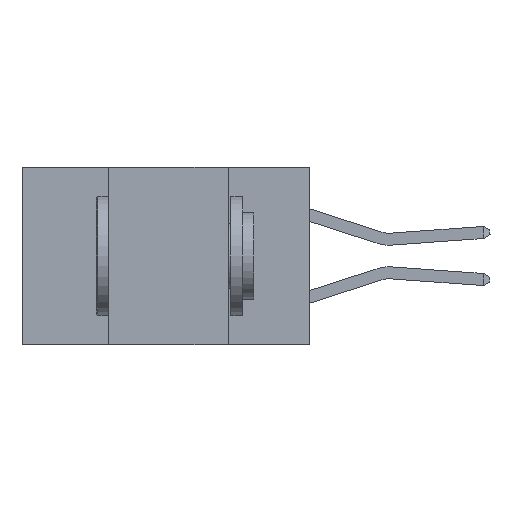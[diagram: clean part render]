
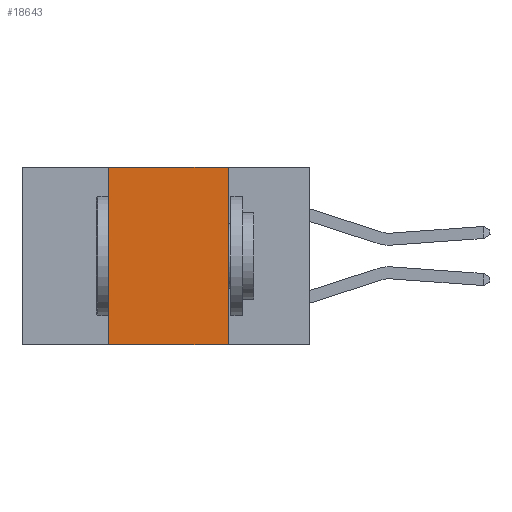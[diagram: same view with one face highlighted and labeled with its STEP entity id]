
A CAD part, left-side view. The second image highlights one B-rep face of the part: STEP entity #18643.
In plain terms, the highlighted planar face has unit normal (-1, 0, 0).
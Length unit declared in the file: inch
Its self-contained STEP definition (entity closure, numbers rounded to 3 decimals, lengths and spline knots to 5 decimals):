
#497 = ORIENTED_EDGE ( 'NONE', *, *, #518, .F. ) ;
#518 = EDGE_CURVE ( 'NONE', #4968, #32732, #17032, .T. ) ;
#2353 = DIRECTION ( 'NONE',  ( 0., 0., -1. ) ) ;
#3965 = VECTOR ( 'NONE', #21358, 39.37008 ) ;
#4008 = EDGE_LOOP ( 'NONE', ( #28634, #497, #12691, #19576 ) ) ;
#4880 = CARTESIAN_POINT ( 'NONE',  ( 0., 0.17, 0. ) ) ;
#4968 = VERTEX_POINT ( 'NONE', #7641 ) ;
#5477 = EDGE_CURVE ( 'NONE', #16546, #4968, #24259, .T. ) ;
#7457 = DIRECTION ( 'NONE',  ( 0., 0., -1. ) ) ;
#7641 = CARTESIAN_POINT ( 'NONE',  ( 0., 0.42, 0. ) ) ;
#9097 = DIRECTION ( 'NONE',  ( 0., -1., 0. ) ) ;
#11531 = FACE_OUTER_BOUND ( 'NONE', #4008, .T. ) ;
#11807 = VERTEX_POINT ( 'NONE', #25793 ) ;
#12496 = VECTOR ( 'NONE', #7457, 39.37008 ) ;
#12691 = ORIENTED_EDGE ( 'NONE', *, *, #5477, .F. ) ;
#13580 = EDGE_CURVE ( 'NONE', #32732, #11807, #26743, .T. ) ;
#14235 = AXIS2_PLACEMENT_3D ( 'NONE', #32670, #17642, #2353 ) ;
#14418 = CARTESIAN_POINT ( 'NONE',  ( 0., 0.6, 0. ) ) ;
#15072 = PLANE ( 'NONE',  #14235 ) ;
#16546 = VERTEX_POINT ( 'NONE', #20273 ) ;
#17032 = LINE ( 'NONE', #14418, #29595 ) ;
#17642 = DIRECTION ( 'NONE',  ( 1., 0., 0. ) ) ;
#18569 = CARTESIAN_POINT ( 'NONE',  ( 0., 0.17, 0. ) ) ;
#18643 = ADVANCED_FACE ( 'NONE', ( #11531 ), #15072, .F. ) ;
#19576 = ORIENTED_EDGE ( 'NONE', *, *, #24811, .T. ) ;
#20273 = CARTESIAN_POINT ( 'NONE',  ( 0., 0.42, -0.37 ) ) ;
#21358 = DIRECTION ( 'NONE',  ( 0., 0., 1. ) ) ;
#23052 = LINE ( 'NONE', #29310, #28893 ) ;
#24259 = LINE ( 'NONE', #27487, #3965 ) ;
#24811 = EDGE_CURVE ( 'NONE', #16546, #11807, #23052, .T. ) ;
#25793 = CARTESIAN_POINT ( 'NONE',  ( 0., 0.17, -0.37 ) ) ;
#26743 = LINE ( 'NONE', #4880, #12496 ) ;
#27487 = CARTESIAN_POINT ( 'NONE',  ( 0., 0.42, 0. ) ) ;
#28634 = ORIENTED_EDGE ( 'NONE', *, *, #13580, .F. ) ;
#28893 = VECTOR ( 'NONE', #9097, 39.37008 ) ;
#29310 = CARTESIAN_POINT ( 'NONE',  ( 0., 0.6, -0.37 ) ) ;
#29480 = DIRECTION ( 'NONE',  ( 0., -1., 0. ) ) ;
#29595 = VECTOR ( 'NONE', #29480, 39.37008 ) ;
#32670 = CARTESIAN_POINT ( 'NONE',  ( 0., 0.6, 0. ) ) ;
#32732 = VERTEX_POINT ( 'NONE', #18569 ) ;
